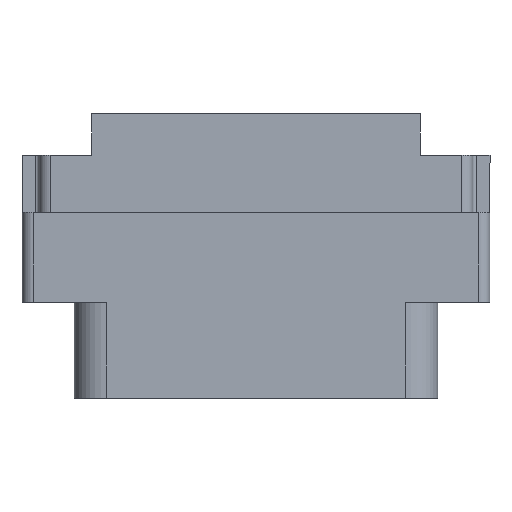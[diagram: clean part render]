
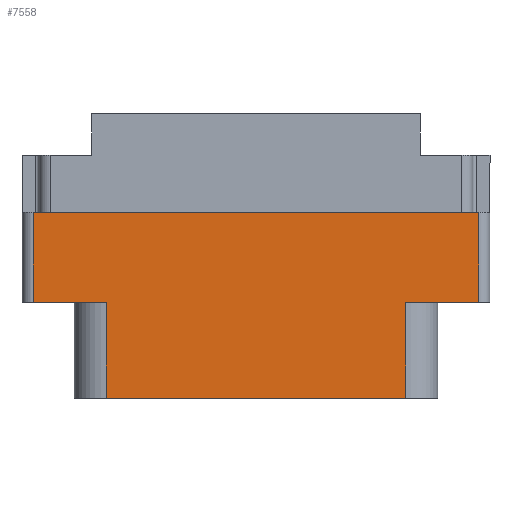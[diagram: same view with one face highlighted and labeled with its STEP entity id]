
A CAD part, front view. The second image highlights one B-rep face of the part: STEP entity #7558.
In plain terms, the highlighted planar face has unit normal (0, -1, 0).
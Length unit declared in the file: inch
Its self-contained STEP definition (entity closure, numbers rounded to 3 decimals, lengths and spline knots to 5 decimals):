
#113 = ORIENTED_EDGE ( 'NONE', *, *, #14529, .T. ) ;
#115 = VECTOR ( 'NONE', #12512, 39.37008 ) ;
#137 = FACE_OUTER_BOUND ( 'NONE', #2589, .T. ) ;
#917 = CARTESIAN_POINT ( 'NONE',  ( -0.656, -0.343, -0.277 ) ) ;
#1052 = CARTESIAN_POINT ( 'NONE',  ( -0.42, -0.343, -0.529 ) ) ;
#1093 = LINE ( 'NONE', #6024, #13617 ) ;
#1677 = CARTESIAN_POINT ( 'NONE',  ( 0.42, -0.343, -0.529 ) ) ;
#1764 = DIRECTION ( 'NONE',  ( 0., 0., -1. ) ) ;
#2119 = ORIENTED_EDGE ( 'NONE', *, *, #13871, .F. ) ;
#2130 = VERTEX_POINT ( 'NONE', #1052 ) ;
#2412 = EDGE_CURVE ( 'NONE', #2130, #20704, #20354, .T. ) ;
#2419 = DIRECTION ( 'NONE',  ( 1., 0., 0. ) ) ;
#2589 = EDGE_LOOP ( 'NONE', ( #10571, #113, #12165, #14948, #11463, #7367, #2119, #21009 ) ) ;
#2595 = LINE ( 'NONE', #12239, #13577 ) ;
#2628 = CARTESIAN_POINT ( 'NONE',  ( -0.624, -0.343, -0.277 ) ) ;
#2716 = VERTEX_POINT ( 'NONE', #1677 ) ;
#2792 = VECTOR ( 'NONE', #2419, 39.37008 ) ;
#3573 = VECTOR ( 'NONE', #14827, 39.37008 ) ;
#4024 = PLANE ( 'NONE',  #11074 ) ;
#5023 = VECTOR ( 'NONE', #7259, 39.37008 ) ;
#5473 = CARTESIAN_POINT ( 'NONE',  ( 0., -0.343, -0.529 ) ) ;
#5496 = VERTEX_POINT ( 'NONE', #11919 ) ;
#6024 = CARTESIAN_POINT ( 'NONE',  ( 0., -0.343, -0.529 ) ) ;
#6393 = EDGE_CURVE ( 'NONE', #13444, #2716, #20053, .T. ) ;
#7204 = EDGE_CURVE ( 'NONE', #2716, #5496, #11178, .T. ) ;
#7230 = VERTEX_POINT ( 'NONE', #18452 ) ;
#7259 = DIRECTION ( 'NONE',  ( 0., 0., -1. ) ) ;
#7367 = ORIENTED_EDGE ( 'NONE', *, *, #19274, .F. ) ;
#7558 = ADVANCED_FACE ( 'NONE', ( #137 ), #4024, .T. ) ;
#7860 = EDGE_CURVE ( 'NONE', #13444, #21020, #8579, .T. ) ;
#8459 = LINE ( 'NONE', #15302, #11295 ) ;
#8570 = CARTESIAN_POINT ( 'NONE',  ( 0.624, -0.343, -0.529 ) ) ;
#8579 = LINE ( 'NONE', #20700, #115 ) ;
#9420 = VECTOR ( 'NONE', #16891, 39.37008 ) ;
#9792 = CARTESIAN_POINT ( 'NONE',  ( -0.42, -0.343, -0.529 ) ) ;
#10571 = ORIENTED_EDGE ( 'NONE', *, *, #2412, .T. ) ;
#10596 = CARTESIAN_POINT ( 'NONE',  ( 0.42, -0.343, -0.529 ) ) ;
#10713 = DIRECTION ( 'NONE',  ( 0., 0., 1. ) ) ;
#11074 = AXIS2_PLACEMENT_3D ( 'NONE', #15468, #19519, #1764 ) ;
#11178 = LINE ( 'NONE', #10596, #5023 ) ;
#11295 = VECTOR ( 'NONE', #10713, 39.37008 ) ;
#11463 = ORIENTED_EDGE ( 'NONE', *, *, #7860, .T. ) ;
#11919 = CARTESIAN_POINT ( 'NONE',  ( 0.42, -0.343, -0.798 ) ) ;
#12109 = VERTEX_POINT ( 'NONE', #2628 ) ;
#12165 = ORIENTED_EDGE ( 'NONE', *, *, #7204, .F. ) ;
#12239 = CARTESIAN_POINT ( 'NONE',  ( -0.624, -0.343, -0.798 ) ) ;
#12512 = DIRECTION ( 'NONE',  ( 0., 0., 1. ) ) ;
#12773 = EDGE_CURVE ( 'NONE', #7230, #2130, #1093, .T. ) ;
#13444 = VERTEX_POINT ( 'NONE', #8570 ) ;
#13577 = VECTOR ( 'NONE', #17349, 39.37008 ) ;
#13617 = VECTOR ( 'NONE', #14379, 39.37008 ) ;
#13871 = EDGE_CURVE ( 'NONE', #7230, #12109, #8459, .T. ) ;
#14379 = DIRECTION ( 'NONE',  ( 1., 0., 0. ) ) ;
#14529 = EDGE_CURVE ( 'NONE', #20704, #5496, #2595, .T. ) ;
#14765 = CARTESIAN_POINT ( 'NONE',  ( -0.42, -0.343, -0.798 ) ) ;
#14827 = DIRECTION ( 'NONE',  ( 0., 0., -1. ) ) ;
#14948 = ORIENTED_EDGE ( 'NONE', *, *, #6393, .F. ) ;
#15302 = CARTESIAN_POINT ( 'NONE',  ( -0.624, -0.343, -0.798 ) ) ;
#15468 = CARTESIAN_POINT ( 'NONE',  ( -0.624, -0.343, -0.798 ) ) ;
#15577 = LINE ( 'NONE', #917, #2792 ) ;
#16891 = DIRECTION ( 'NONE',  ( -1., 0., 0. ) ) ;
#17349 = DIRECTION ( 'NONE',  ( 1., 0., 0. ) ) ;
#18452 = CARTESIAN_POINT ( 'NONE',  ( -0.624, -0.343, -0.529 ) ) ;
#19274 = EDGE_CURVE ( 'NONE', #12109, #21020, #15577, .T. ) ;
#19519 = DIRECTION ( 'NONE',  ( 0., -1., 0. ) ) ;
#20053 = LINE ( 'NONE', #5473, #9420 ) ;
#20354 = LINE ( 'NONE', #9792, #3573 ) ;
#20700 = CARTESIAN_POINT ( 'NONE',  ( 0.624, -0.343, -0.798 ) ) ;
#20704 = VERTEX_POINT ( 'NONE', #14765 ) ;
#20829 = CARTESIAN_POINT ( 'NONE',  ( 0.624, -0.343, -0.277 ) ) ;
#21009 = ORIENTED_EDGE ( 'NONE', *, *, #12773, .T. ) ;
#21020 = VERTEX_POINT ( 'NONE', #20829 ) ;
